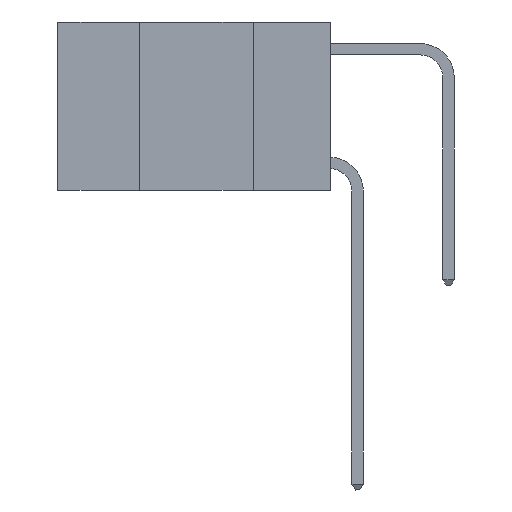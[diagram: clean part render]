
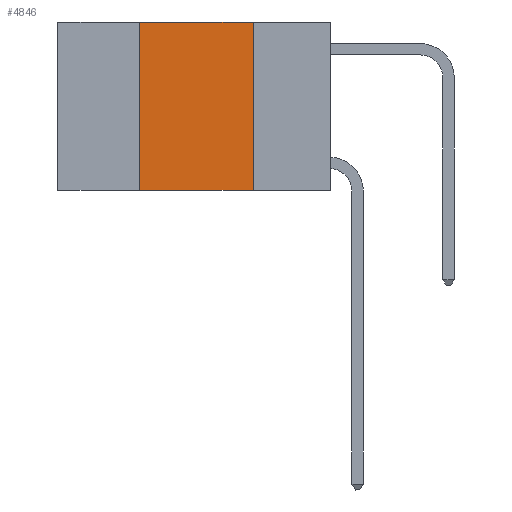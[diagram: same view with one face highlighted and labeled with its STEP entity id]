
A CAD part, left-side view. The second image highlights one B-rep face of the part: STEP entity #4846.
In plain terms, the highlighted planar face has unit normal (-1, 0, 0).
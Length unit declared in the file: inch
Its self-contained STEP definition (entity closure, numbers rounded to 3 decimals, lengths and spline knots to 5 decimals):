
#169 = CARTESIAN_POINT ( 'NONE',  ( 0., 0.42, 0. ) ) ;
#174 = FACE_OUTER_BOUND ( 'NONE', #180, .T. ) ;
#180 = EDGE_LOOP ( 'NONE', ( #15351, #8441, #14049, #5432 ) ) ;
#467 = LINE ( 'NONE', #5865, #10257 ) ;
#1933 = VERTEX_POINT ( 'NONE', #14904 ) ;
#3328 = VERTEX_POINT ( 'NONE', #11094 ) ;
#3627 = VECTOR ( 'NONE', #13114, 39.37008 ) ;
#3969 = DIRECTION ( 'NONE',  ( 0., 0., -1. ) ) ;
#4091 = DIRECTION ( 'NONE',  ( 0., 0., -1. ) ) ;
#4266 = EDGE_CURVE ( 'NONE', #11905, #3328, #467, .T. ) ;
#4788 = AXIS2_PLACEMENT_3D ( 'NONE', #5408, #5242, #3969 ) ;
#4846 = ADVANCED_FACE ( 'NONE', ( #174 ), #9307, .F. ) ;
#5242 = DIRECTION ( 'NONE',  ( 1., 0., 0. ) ) ;
#5257 = VECTOR ( 'NONE', #4091, 39.37008 ) ;
#5408 = CARTESIAN_POINT ( 'NONE',  ( 0., 0.6, 0. ) ) ;
#5432 = ORIENTED_EDGE ( 'NONE', *, *, #6074, .T. ) ;
#5865 = CARTESIAN_POINT ( 'NONE',  ( 0., 0.6, 0. ) ) ;
#6074 = EDGE_CURVE ( 'NONE', #11885, #1933, #6754, .T. ) ;
#6754 = LINE ( 'NONE', #14393, #12223 ) ;
#8441 = ORIENTED_EDGE ( 'NONE', *, *, #4266, .F. ) ;
#8916 = EDGE_CURVE ( 'NONE', #11885, #11905, #9465, .T. ) ;
#9307 = PLANE ( 'NONE',  #4788 ) ;
#9348 = LINE ( 'NONE', #10698, #5257 ) ;
#9465 = LINE ( 'NONE', #169, #3627 ) ;
#9757 = CARTESIAN_POINT ( 'NONE',  ( 0., 0.42, 0. ) ) ;
#10257 = VECTOR ( 'NONE', #13586, 39.37008 ) ;
#10554 = EDGE_CURVE ( 'NONE', #3328, #1933, #9348, .T. ) ;
#10698 = CARTESIAN_POINT ( 'NONE',  ( 0., 0.17, 0. ) ) ;
#11094 = CARTESIAN_POINT ( 'NONE',  ( 0., 0.17, 0. ) ) ;
#11885 = VERTEX_POINT ( 'NONE', #13587 ) ;
#11905 = VERTEX_POINT ( 'NONE', #9757 ) ;
#12223 = VECTOR ( 'NONE', #15836, 39.37008 ) ;
#13114 = DIRECTION ( 'NONE',  ( 0., 0., 1. ) ) ;
#13586 = DIRECTION ( 'NONE',  ( 0., -1., 0. ) ) ;
#13587 = CARTESIAN_POINT ( 'NONE',  ( 0., 0.42, -0.37 ) ) ;
#14049 = ORIENTED_EDGE ( 'NONE', *, *, #8916, .F. ) ;
#14393 = CARTESIAN_POINT ( 'NONE',  ( 0., 0.6, -0.37 ) ) ;
#14904 = CARTESIAN_POINT ( 'NONE',  ( 0., 0.17, -0.37 ) ) ;
#15351 = ORIENTED_EDGE ( 'NONE', *, *, #10554, .F. ) ;
#15836 = DIRECTION ( 'NONE',  ( 0., -1., 0. ) ) ;
